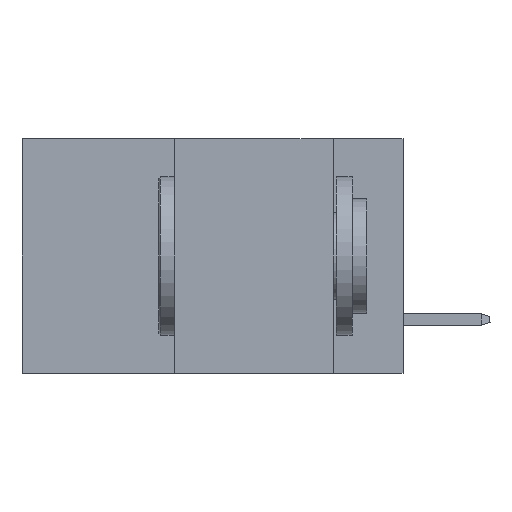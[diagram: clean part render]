
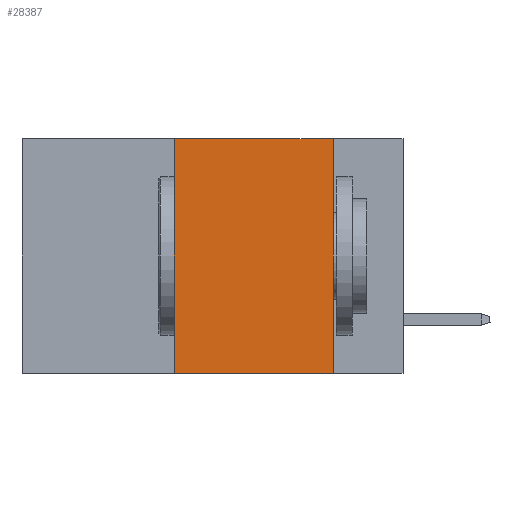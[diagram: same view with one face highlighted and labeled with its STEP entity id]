
A CAD part, left-side view. The second image highlights one B-rep face of the part: STEP entity #28387.
In plain terms, the highlighted planar face has unit normal (-1, 0, 0).
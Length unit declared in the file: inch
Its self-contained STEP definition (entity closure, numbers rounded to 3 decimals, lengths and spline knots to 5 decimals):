
#235 = EDGE_LOOP ( 'NONE', ( #14645, #28692, #18734, #6730 ) ) ;
#1084 = CARTESIAN_POINT ( 'NONE',  ( 0., 0.6, 0. ) ) ;
#1864 = VECTOR ( 'NONE', #18778, 39.37008 ) ;
#2644 = AXIS2_PLACEMENT_3D ( 'NONE', #30814, #23656, #16944 ) ;
#4656 = CARTESIAN_POINT ( 'NONE',  ( 0., 0.11, 0. ) ) ;
#5903 = VERTEX_POINT ( 'NONE', #7480 ) ;
#6247 = DIRECTION ( 'NONE',  ( 0., -1., 0. ) ) ;
#6730 = ORIENTED_EDGE ( 'NONE', *, *, #29064, .T. ) ;
#6865 = VECTOR ( 'NONE', #6247, 39.37008 ) ;
#7480 = CARTESIAN_POINT ( 'NONE',  ( 0., 0.36, 0. ) ) ;
#7591 = VECTOR ( 'NONE', #39536, 39.37008 ) ;
#9542 = FACE_OUTER_BOUND ( 'NONE', #235, .T. ) ;
#9856 = LINE ( 'NONE', #13016, #28513 ) ;
#12622 = EDGE_CURVE ( 'NONE', #37543, #5903, #9856, .T. ) ;
#13016 = CARTESIAN_POINT ( 'NONE',  ( 0., 0.36, 0. ) ) ;
#14645 = ORIENTED_EDGE ( 'NONE', *, *, #29528, .F. ) ;
#16944 = DIRECTION ( 'NONE',  ( 0., 0., -1. ) ) ;
#18076 = VERTEX_POINT ( 'NONE', #4656 ) ;
#18734 = ORIENTED_EDGE ( 'NONE', *, *, #12622, .F. ) ;
#18778 = DIRECTION ( 'NONE',  ( 0., -1., 0. ) ) ;
#18979 = LINE ( 'NONE', #29718, #7591 ) ;
#21340 = PLANE ( 'NONE',  #2644 ) ;
#23205 = VERTEX_POINT ( 'NONE', #40141 ) ;
#23656 = DIRECTION ( 'NONE',  ( 1., 0., 0. ) ) ;
#26859 = LINE ( 'NONE', #39585, #6865 ) ;
#28387 = ADVANCED_FACE ( 'NONE', ( #9542 ), #21340, .F. ) ;
#28513 = VECTOR ( 'NONE', #43654, 39.37008 ) ;
#28692 = ORIENTED_EDGE ( 'NONE', *, *, #29411, .F. ) ;
#29064 = EDGE_CURVE ( 'NONE', #37543, #23205, #26859, .T. ) ;
#29411 = EDGE_CURVE ( 'NONE', #5903, #18076, #38874, .T. ) ;
#29528 = EDGE_CURVE ( 'NONE', #18076, #23205, #18979, .T. ) ;
#29718 = CARTESIAN_POINT ( 'NONE',  ( 0., 0.11, 0. ) ) ;
#29964 = CARTESIAN_POINT ( 'NONE',  ( 0., 0.36, -0.37 ) ) ;
#30814 = CARTESIAN_POINT ( 'NONE',  ( 0., 0.6, 0. ) ) ;
#37543 = VERTEX_POINT ( 'NONE', #29964 ) ;
#38874 = LINE ( 'NONE', #1084, #1864 ) ;
#39536 = DIRECTION ( 'NONE',  ( 0., 0., -1. ) ) ;
#39585 = CARTESIAN_POINT ( 'NONE',  ( 0., 0.6, -0.37 ) ) ;
#40141 = CARTESIAN_POINT ( 'NONE',  ( 0., 0.11, -0.37 ) ) ;
#43654 = DIRECTION ( 'NONE',  ( 0., 0., 1. ) ) ;
